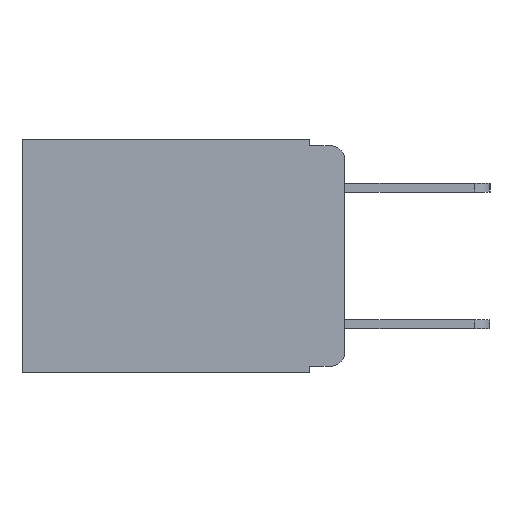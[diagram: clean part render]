
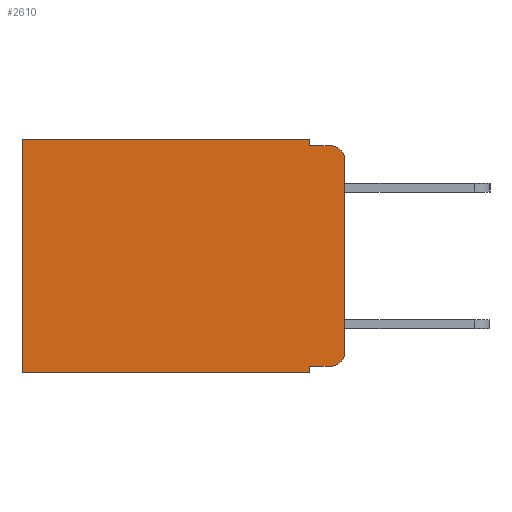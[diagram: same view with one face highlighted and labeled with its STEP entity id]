
A CAD part, left-side view. The second image highlights one B-rep face of the part: STEP entity #2610.
In plain terms, the highlighted planar face has unit normal (-1, 0, 0).
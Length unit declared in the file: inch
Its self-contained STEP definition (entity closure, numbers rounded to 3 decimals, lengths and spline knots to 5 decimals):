
#17 = AXIS2_PLACEMENT_3D ( 'NONE', #10495, #4364, #11426 ) ;
#112 = LINE ( 'NONE', #11049, #11362 ) ;
#222 = DIRECTION ( 'NONE',  ( -1., 0., 0. ) ) ;
#558 = ORIENTED_EDGE ( 'NONE', *, *, #10344, .F. ) ;
#623 = DIRECTION ( 'NONE',  ( 0., 0., -1. ) ) ;
#717 = PLANE ( 'NONE',  #5363 ) ;
#829 = CARTESIAN_POINT ( 'NONE',  ( 0.298, 0.473, -0.343 ) ) ;
#1059 = VERTEX_POINT ( 'NONE', #9707 ) ;
#1160 = VECTOR ( 'NONE', #7052, 39.37008 ) ;
#1286 = ORIENTED_EDGE ( 'NONE', *, *, #9245, .F. ) ;
#1326 = CARTESIAN_POINT ( 'NONE',  ( 0.298, 0.473, 0. ) ) ;
#1585 = LINE ( 'NONE', #1326, #1160 ) ;
#1757 = CARTESIAN_POINT ( 'NONE',  ( 0.298, 0., 0. ) ) ;
#1799 = VERTEX_POINT ( 'NONE', #5291 ) ;
#1807 = ORIENTED_EDGE ( 'NONE', *, *, #9735, .T. ) ;
#1810 = VERTEX_POINT ( 'NONE', #10286 ) ;
#1817 = DIRECTION ( 'NONE',  ( 0., 1., 0. ) ) ;
#1864 = CARTESIAN_POINT ( 'NONE',  ( 0.298, 0.02, -0.01 ) ) ;
#1959 = CARTESIAN_POINT ( 'NONE',  ( 0.298, 0., 0. ) ) ;
#2001 = ORIENTED_EDGE ( 'NONE', *, *, #8429, .T. ) ;
#2007 = VERTEX_POINT ( 'NONE', #5456 ) ;
#2031 = ORIENTED_EDGE ( 'NONE', *, *, #10957, .F. ) ;
#2034 = DIRECTION ( 'NONE',  ( 0., -1., 0. ) ) ;
#2072 = ORIENTED_EDGE ( 'NONE', *, *, #9082, .F. ) ;
#2278 = ORIENTED_EDGE ( 'NONE', *, *, #13387, .F. ) ;
#2610 = ADVANCED_FACE ( 'NONE', ( #10972 ), #717, .F. ) ;
#2671 = ORIENTED_EDGE ( 'NONE', *, *, #7737, .T. ) ;
#3101 = AXIS2_PLACEMENT_3D ( 'NONE', #7246, #222, #8280 ) ;
#3567 = DIRECTION ( 'NONE',  ( 0., 0., -1. ) ) ;
#3570 = VECTOR ( 'NONE', #623, 39.37008 ) ;
#3950 = LINE ( 'NONE', #13186, #3570 ) ;
#4234 = VERTEX_POINT ( 'NONE', #5168 ) ;
#4364 = DIRECTION ( 'NONE',  ( -1., 0., 0. ) ) ;
#4439 = EDGE_CURVE ( 'NONE', #1810, #7574, #6947, .T. ) ;
#4453 = VERTEX_POINT ( 'NONE', #1864 ) ;
#4754 = EDGE_LOOP ( 'NONE', ( #2278, #5541, #2031, #558, #6074, #1807, #1286, #2072, #2001, #2671 ) ) ;
#4900 = VECTOR ( 'NONE', #7931, 39.37008 ) ;
#5027 = DIRECTION ( 'NONE',  ( 0., 0., -1. ) ) ;
#5090 = LINE ( 'NONE', #8460, #9936 ) ;
#5168 = CARTESIAN_POINT ( 'NONE',  ( 0.298, 0.051, -0.343 ) ) ;
#5282 = DIRECTION ( 'NONE',  ( 0., -1., 0. ) ) ;
#5291 = CARTESIAN_POINT ( 'NONE',  ( 0.298, 0., -0.313 ) ) ;
#5363 = AXIS2_PLACEMENT_3D ( 'NONE', #1959, #10823, #3567 ) ;
#5456 = CARTESIAN_POINT ( 'NONE',  ( 0.298, 0.02, -0.333 ) ) ;
#5541 = ORIENTED_EDGE ( 'NONE', *, *, #11574, .T. ) ;
#6074 = ORIENTED_EDGE ( 'NONE', *, *, #4439, .T. ) ;
#6647 = VECTOR ( 'NONE', #8410, 39.37008 ) ;
#6947 = LINE ( 'NONE', #1757, #6647 ) ;
#7052 = DIRECTION ( 'NONE',  ( 0., 0., -1. ) ) ;
#7100 = VERTEX_POINT ( 'NONE', #829 ) ;
#7246 = CARTESIAN_POINT ( 'NONE',  ( 0.298, 0.02, -0.03 ) ) ;
#7574 = VERTEX_POINT ( 'NONE', #13025 ) ;
#7737 = EDGE_CURVE ( 'NONE', #2007, #1799, #8926, .T. ) ;
#7742 = LINE ( 'NONE', #10800, #4900 ) ;
#7931 = DIRECTION ( 'NONE',  ( 0., 0., -1. ) ) ;
#8254 = CARTESIAN_POINT ( 'NONE',  ( 0.298, 0.051, -0.01 ) ) ;
#8280 = DIRECTION ( 'NONE',  ( 0., 0., -1. ) ) ;
#8410 = DIRECTION ( 'NONE',  ( 0., 1., 0. ) ) ;
#8429 = EDGE_CURVE ( 'NONE', #9669, #2007, #11528, .T. ) ;
#8460 = CARTESIAN_POINT ( 'NONE',  ( 0.298, 0., -0.343 ) ) ;
#8627 = CARTESIAN_POINT ( 'NONE',  ( 0.298, 0.051, -0.333 ) ) ;
#8859 = VERTEX_POINT ( 'NONE', #8254 ) ;
#8926 = CIRCLE ( 'NONE', #17, 0.02 ) ;
#9082 = EDGE_CURVE ( 'NONE', #9669, #4234, #112, .T. ) ;
#9245 = EDGE_CURVE ( 'NONE', #4234, #7100, #5090, .T. ) ;
#9353 = VECTOR ( 'NONE', #2034, 39.37008 ) ;
#9669 = VERTEX_POINT ( 'NONE', #12657 ) ;
#9707 = CARTESIAN_POINT ( 'NONE',  ( 0.298, 0., -0.03 ) ) ;
#9735 = EDGE_CURVE ( 'NONE', #7574, #7100, #1585, .T. ) ;
#9886 = VECTOR ( 'NONE', #5282, 39.37008 ) ;
#9936 = VECTOR ( 'NONE', #1817, 39.37008 ) ;
#10286 = CARTESIAN_POINT ( 'NONE',  ( 0.298, 0.051, 0. ) ) ;
#10344 = EDGE_CURVE ( 'NONE', #1810, #8859, #7742, .T. ) ;
#10495 = CARTESIAN_POINT ( 'NONE',  ( 0.298, 0.02, -0.313 ) ) ;
#10800 = CARTESIAN_POINT ( 'NONE',  ( 0.298, 0.051, 0. ) ) ;
#10823 = DIRECTION ( 'NONE',  ( 1., 0., 0. ) ) ;
#10957 = EDGE_CURVE ( 'NONE', #8859, #4453, #12292, .T. ) ;
#10972 = FACE_OUTER_BOUND ( 'NONE', #4754, .T. ) ;
#11049 = CARTESIAN_POINT ( 'NONE',  ( 0.298, 0.051, 0. ) ) ;
#11362 = VECTOR ( 'NONE', #5027, 39.37008 ) ;
#11426 = DIRECTION ( 'NONE',  ( 0., 0., -1. ) ) ;
#11528 = LINE ( 'NONE', #8627, #9353 ) ;
#11574 = EDGE_CURVE ( 'NONE', #1059, #4453, #13276, .T. ) ;
#12151 = CARTESIAN_POINT ( 'NONE',  ( 0.298, 0.051, -0.01 ) ) ;
#12292 = LINE ( 'NONE', #12151, #9886 ) ;
#12657 = CARTESIAN_POINT ( 'NONE',  ( 0.298, 0.051, -0.333 ) ) ;
#13025 = CARTESIAN_POINT ( 'NONE',  ( 0.298, 0.473, 0. ) ) ;
#13186 = CARTESIAN_POINT ( 'NONE',  ( 0.298, 0., 0. ) ) ;
#13276 = CIRCLE ( 'NONE', #3101, 0.02 ) ;
#13387 = EDGE_CURVE ( 'NONE', #1059, #1799, #3950, .T. ) ;
